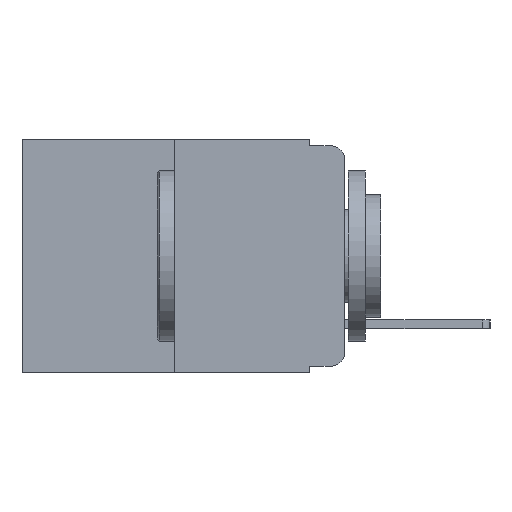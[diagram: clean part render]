
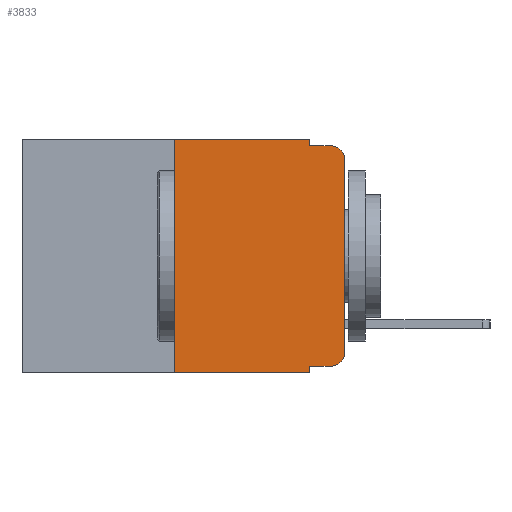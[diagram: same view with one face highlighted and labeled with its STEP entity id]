
A CAD part, left-side view. The second image highlights one B-rep face of the part: STEP entity #3833.
In plain terms, the highlighted planar face has unit normal (-1, 0, 0).
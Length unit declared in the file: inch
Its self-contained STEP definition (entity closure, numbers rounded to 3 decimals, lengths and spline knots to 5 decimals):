
#92 = CIRCLE ( 'NONE', #19475, 0.02 ) ;
#120 = DIRECTION ( 'NONE',  ( 0., -1., 0. ) ) ;
#1157 = AXIS2_PLACEMENT_3D ( 'NONE', #13940, #8370, #9735 ) ;
#1262 = LINE ( 'NONE', #13690, #21274 ) ;
#1412 = VECTOR ( 'NONE', #20817, 39.37008 ) ;
#1988 = CARTESIAN_POINT ( 'NONE',  ( 0., 0.051, 0. ) ) ;
#2163 = DIRECTION ( 'NONE',  ( 0., 0., 1. ) ) ;
#2321 = DIRECTION ( 'NONE',  ( -1., 0., 0. ) ) ;
#2419 = ORIENTED_EDGE ( 'NONE', *, *, #23884, .F. ) ;
#3407 = VERTEX_POINT ( 'NONE', #17649 ) ;
#3833 = ADVANCED_FACE ( 'NONE', ( #21756 ), #19529, .F. ) ;
#4005 = CARTESIAN_POINT ( 'NONE',  ( 0., 0.051, 0. ) ) ;
#4023 = LINE ( 'NONE', #19766, #14223 ) ;
#4168 = VERTEX_POINT ( 'NONE', #1988 ) ;
#4619 = CARTESIAN_POINT ( 'NONE',  ( 0., 0.051, -0.01 ) ) ;
#4694 = CARTESIAN_POINT ( 'NONE',  ( 0., 0., -0.03 ) ) ;
#5794 = ORIENTED_EDGE ( 'NONE', *, *, #20028, .F. ) ;
#5870 = AXIS2_PLACEMENT_3D ( 'NONE', #17592, #6350, #19378 ) ;
#6124 = ORIENTED_EDGE ( 'NONE', *, *, #17965, .T. ) ;
#6350 = DIRECTION ( 'NONE',  ( -1., 0., 0. ) ) ;
#6537 = CARTESIAN_POINT ( 'NONE',  ( 0., 0.25, -0.343 ) ) ;
#6564 = DIRECTION ( 'NONE',  ( 0., -1., 0. ) ) ;
#6752 = VERTEX_POINT ( 'NONE', #16259 ) ;
#6916 = VECTOR ( 'NONE', #6564, 39.37008 ) ;
#7047 = VERTEX_POINT ( 'NONE', #22496 ) ;
#7086 = CARTESIAN_POINT ( 'NONE',  ( 0., 0.051, -0.333 ) ) ;
#7329 = ORIENTED_EDGE ( 'NONE', *, *, #15281, .F. ) ;
#7370 = LINE ( 'NONE', #4005, #13053 ) ;
#7473 = VERTEX_POINT ( 'NONE', #14638 ) ;
#7940 = CARTESIAN_POINT ( 'NONE',  ( 0., 0., 0. ) ) ;
#8224 = ORIENTED_EDGE ( 'NONE', *, *, #16473, .F. ) ;
#8370 = DIRECTION ( 'NONE',  ( 1., 0., 0. ) ) ;
#8651 = CARTESIAN_POINT ( 'NONE',  ( 0., 0.473, -0.343 ) ) ;
#8734 = DIRECTION ( 'NONE',  ( 0., 0., -1. ) ) ;
#9196 = VERTEX_POINT ( 'NONE', #15998 ) ;
#9735 = DIRECTION ( 'NONE',  ( 0., 0., -1. ) ) ;
#10236 = EDGE_CURVE ( 'NONE', #9196, #6752, #92, .T. ) ;
#10367 = LINE ( 'NONE', #8651, #14784 ) ;
#11748 = LINE ( 'NONE', #7940, #1412 ) ;
#12121 = ORIENTED_EDGE ( 'NONE', *, *, #17668, .F. ) ;
#12337 = VERTEX_POINT ( 'NONE', #4619 ) ;
#12426 = ORIENTED_EDGE ( 'NONE', *, *, #14038, .T. ) ;
#12640 = LINE ( 'NONE', #16005, #6916 ) ;
#13034 = VERTEX_POINT ( 'NONE', #6537 ) ;
#13053 = VECTOR ( 'NONE', #19003, 39.37008 ) ;
#13690 = CARTESIAN_POINT ( 'NONE',  ( 0., 0.051, -0.01 ) ) ;
#13809 = VERTEX_POINT ( 'NONE', #17721 ) ;
#13874 = CARTESIAN_POINT ( 'NONE',  ( 0., 0.02, -0.313 ) ) ;
#13940 = CARTESIAN_POINT ( 'NONE',  ( 0., 0.473, 0. ) ) ;
#14038 = EDGE_CURVE ( 'NONE', #7047, #9196, #18502, .T. ) ;
#14223 = VECTOR ( 'NONE', #8734, 39.37008 ) ;
#14490 = LINE ( 'NONE', #15581, #18668 ) ;
#14638 = CARTESIAN_POINT ( 'NONE',  ( 0., 0.051, -0.343 ) ) ;
#14747 = ORIENTED_EDGE ( 'NONE', *, *, #23701, .T. ) ;
#14784 = VECTOR ( 'NONE', #19685, 39.37008 ) ;
#14885 = EDGE_LOOP ( 'NONE', ( #14747, #19488, #5794, #12121, #2419, #8224, #6124, #7329, #12426, #24327 ) ) ;
#15281 = EDGE_CURVE ( 'NONE', #7047, #7473, #4023, .T. ) ;
#15581 = CARTESIAN_POINT ( 'NONE',  ( 0., 0.25, 0. ) ) ;
#15739 = DIRECTION ( 'NONE',  ( 0., 0., -1. ) ) ;
#15998 = CARTESIAN_POINT ( 'NONE',  ( 0., 0.02, -0.333 ) ) ;
#16005 = CARTESIAN_POINT ( 'NONE',  ( 0., 0.473, 0. ) ) ;
#16259 = CARTESIAN_POINT ( 'NONE',  ( 0., 0., -0.313 ) ) ;
#16473 = EDGE_CURVE ( 'NONE', #13034, #3407, #14490, .T. ) ;
#17592 = CARTESIAN_POINT ( 'NONE',  ( 0., 0.02, -0.03 ) ) ;
#17649 = CARTESIAN_POINT ( 'NONE',  ( 0., 0.25, 0. ) ) ;
#17668 = EDGE_CURVE ( 'NONE', #4168, #12337, #7370, .T. ) ;
#17721 = CARTESIAN_POINT ( 'NONE',  ( 0., 0.02, -0.01 ) ) ;
#17946 = VECTOR ( 'NONE', #20108, 39.37008 ) ;
#17965 = EDGE_CURVE ( 'NONE', #13034, #7473, #10367, .T. ) ;
#18502 = LINE ( 'NONE', #7086, #17946 ) ;
#18668 = VECTOR ( 'NONE', #2163, 39.37008 ) ;
#19003 = DIRECTION ( 'NONE',  ( 0., 0., -1. ) ) ;
#19378 = DIRECTION ( 'NONE',  ( 0., 0., -1. ) ) ;
#19475 = AXIS2_PLACEMENT_3D ( 'NONE', #13874, #2321, #15739 ) ;
#19488 = ORIENTED_EDGE ( 'NONE', *, *, #22475, .T. ) ;
#19529 = PLANE ( 'NONE',  #1157 ) ;
#19685 = DIRECTION ( 'NONE',  ( 0., -1., 0. ) ) ;
#19766 = CARTESIAN_POINT ( 'NONE',  ( 0., 0.051, 0. ) ) ;
#20028 = EDGE_CURVE ( 'NONE', #12337, #13809, #1262, .T. ) ;
#20108 = DIRECTION ( 'NONE',  ( 0., -1., 0. ) ) ;
#20817 = DIRECTION ( 'NONE',  ( 0., 0., 1. ) ) ;
#21274 = VECTOR ( 'NONE', #120, 39.37008 ) ;
#21756 = FACE_OUTER_BOUND ( 'NONE', #14885, .T. ) ;
#21972 = VERTEX_POINT ( 'NONE', #4694 ) ;
#22475 = EDGE_CURVE ( 'NONE', #21972, #13809, #24279, .T. ) ;
#22496 = CARTESIAN_POINT ( 'NONE',  ( 0., 0.051, -0.333 ) ) ;
#23701 = EDGE_CURVE ( 'NONE', #6752, #21972, #11748, .T. ) ;
#23884 = EDGE_CURVE ( 'NONE', #3407, #4168, #12640, .T. ) ;
#24279 = CIRCLE ( 'NONE', #5870, 0.02 ) ;
#24327 = ORIENTED_EDGE ( 'NONE', *, *, #10236, .T. ) ;
